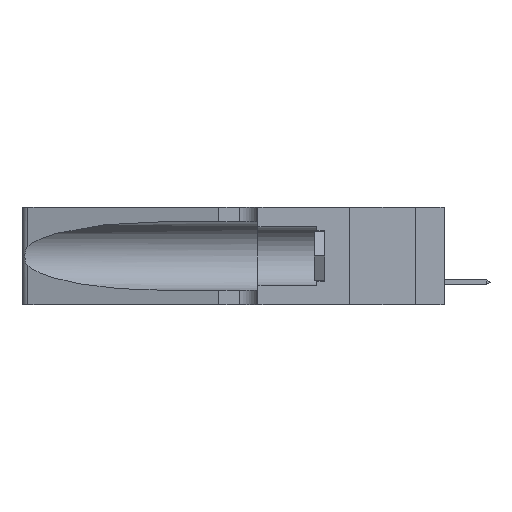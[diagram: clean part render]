
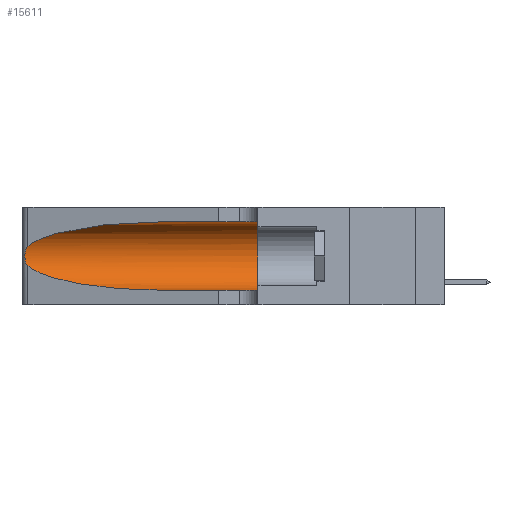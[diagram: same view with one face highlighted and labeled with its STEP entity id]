
A CAD part, left-side view. The second image highlights one B-rep face of the part: STEP entity #15611.
In plain terms, the highlighted cylindrical face has radius 3.308 mm (diameter 6.617 mm), a partial arc.
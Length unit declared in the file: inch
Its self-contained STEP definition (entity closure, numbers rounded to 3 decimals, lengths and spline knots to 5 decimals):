
#83 = B_SPLINE_CURVE_WITH_KNOTS ( 'NONE', 3,
 ( #15689, #11166, #17292, #9687, #17689, #11497, #3763, #14531, #15977, #2344, #2477, #9822, #13083, #13143 ),
 .UNSPECIFIED., .F., .F.,
 ( 4, 2, 2, 2, 2, 2, 4 ),
 ( 0., 0.00027, 0.00053, 0.00107, 0.0016, 0.00187, 0.00214 ),
 .UNSPECIFIED. ) ;
#306 = EDGE_CURVE ( 'NONE', #17060, #13026, #18665, .T. ) ;
#445 = LINE ( 'NONE', #8577, #11906 ) ;
#906 = ORIENTED_EDGE ( 'NONE', *, *, #6104, .T. ) ;
#977 = DIRECTION ( 'NONE',  ( 0., -1., 0. ) ) ;
#1337 = DIRECTION ( 'NONE',  ( 0., 1., 0. ) ) ;
#1874 = EDGE_CURVE ( 'NONE', #13601, #13559, #445, .T. ) ;
#2181 = VECTOR ( 'NONE', #18388, 39.37008 ) ;
#2231 = CIRCLE ( 'NONE', #17281, 0.13025 ) ;
#2344 = CARTESIAN_POINT ( 'NONE',  ( 0.25856, 1.23593, 0.16098 ) ) ;
#2477 = CARTESIAN_POINT ( 'NONE',  ( 0.25789, 1.23486, 0.15765 ) ) ;
#2861 = DIRECTION ( 'NONE',  ( 0., 0., 1. ) ) ;
#3026 =( BOUNDED_CURVE ( )  B_SPLINE_CURVE ( 3, ( #3247, #9378, #3380, #12407 ),
 .UNSPECIFIED., .F., .T. ) 
 B_SPLINE_CURVE_WITH_KNOTS ( ( 4, 4 ),
 ( 3.44316, 4.71239 ),
 .UNSPECIFIED. ) 
 CURVE ( )  GEOMETRIC_REPRESENTATION_ITEM ( )  RATIONAL_B_SPLINE_CURVE ( ( 1., 0.87, 0.87, 1. ) ) 
 REPRESENTATION_ITEM ( '' )  );
#3247 = CARTESIAN_POINT ( 'NONE',  ( 0.25487, 1.22718, 0.14631 ) ) ;
#3380 = CARTESIAN_POINT ( 'NONE',  ( 0.18966, 0.96281, 0.05475 ) ) ;
#3763 = CARTESIAN_POINT ( 'NONE',  ( 0.26075, 1.23896, 0.19203 ) ) ;
#4534 = CARTESIAN_POINT ( 'NONE',  ( 0.1305, 1.61858, 0.31525 ) ) ;
#5158 = EDGE_CURVE ( 'NONE', #13026, #13559, #2231, .T. ) ;
#5350 = CARTESIAN_POINT ( 'NONE',  ( 0.1305, 1.61858, 0.185 ) ) ;
#6104 = EDGE_CURVE ( 'NONE', #9399, #13601, #3026, .T. ) ;
#6399 = EDGE_CURVE ( 'NONE', #17060, #7415, #15752, .T. ) ;
#6512 = CYLINDRICAL_SURFACE ( 'NONE', #12287, 0.13025 ) ;
#6953 = ORIENTED_EDGE ( 'NONE', *, *, #5158, .F. ) ;
#7166 = ORIENTED_EDGE ( 'NONE', *, *, #10112, .T. ) ;
#7371 = CARTESIAN_POINT ( 'NONE',  ( 0.1305, 0.72297, 0.31525 ) ) ;
#7415 = VERTEX_POINT ( 'NONE', #14975 ) ;
#8577 = CARTESIAN_POINT ( 'NONE',  ( 0.1305, 1.61858, 0.05475 ) ) ;
#8954 = ORIENTED_EDGE ( 'NONE', *, *, #6399, .T. ) ;
#9262 = EDGE_LOOP ( 'NONE', ( #8954, #7166, #906, #17290, #6953, #16224 ) ) ;
#9378 = CARTESIAN_POINT ( 'NONE',  ( 0.2373, 1.15595, 0.08982 ) ) ;
#9399 = VERTEX_POINT ( 'NONE', #15605 ) ;
#9687 = CARTESIAN_POINT ( 'NONE',  ( 0.25787, 1.23484, 0.2124 ) ) ;
#9799 = CARTESIAN_POINT ( 'NONE',  ( 0.18966, 0.96281, 0.31525 ) ) ;
#9822 = CARTESIAN_POINT ( 'NONE',  ( 0.25639, 1.23186, 0.15144 ) ) ;
#10112 = EDGE_CURVE ( 'NONE', #7415, #9399, #83, .T. ) ;
#10599 = CARTESIAN_POINT ( 'NONE',  ( 0.1305, 0.35, 0.185 ) ) ;
#11166 = CARTESIAN_POINT ( 'NONE',  ( 0.25555, 1.22994, 0.2215 ) ) ;
#11497 = CARTESIAN_POINT ( 'NONE',  ( 0.26018, 1.23835, 0.19895 ) ) ;
#11552 = DIRECTION ( 'NONE',  ( 0., -1., 0. ) ) ;
#11618 = CARTESIAN_POINT ( 'NONE',  ( 0.1305, 0.72297, 0.05475 ) ) ;
#11877 = CARTESIAN_POINT ( 'NONE',  ( 0.2373, 1.15595, 0.28018 ) ) ;
#11906 = VECTOR ( 'NONE', #977, 39.37008 ) ;
#12287 = AXIS2_PLACEMENT_3D ( 'NONE', #5350, #11552, #18897 ) ;
#12407 = CARTESIAN_POINT ( 'NONE',  ( 0.1305, 0.72297, 0.05475 ) ) ;
#13026 = VERTEX_POINT ( 'NONE', #18769 ) ;
#13083 = CARTESIAN_POINT ( 'NONE',  ( 0.25555, 1.22993, 0.14849 ) ) ;
#13143 = CARTESIAN_POINT ( 'NONE',  ( 0.25487, 1.22718, 0.14631 ) ) ;
#13559 = VERTEX_POINT ( 'NONE', #17091 ) ;
#13601 = VERTEX_POINT ( 'NONE', #11618 ) ;
#14350 = FACE_OUTER_BOUND ( 'NONE', #9262, .T. ) ;
#14531 = CARTESIAN_POINT ( 'NONE',  ( 0.26075, 1.23896, 0.178 ) ) ;
#14975 = CARTESIAN_POINT ( 'NONE',  ( 0.25487, 1.22718, 0.22369 ) ) ;
#15605 = CARTESIAN_POINT ( 'NONE',  ( 0.25487, 1.22718, 0.14631 ) ) ;
#15611 = ADVANCED_FACE ( 'NONE', ( #14350 ), #6512, .F. ) ;
#15689 = CARTESIAN_POINT ( 'NONE',  ( 0.25487, 1.22718, 0.22369 ) ) ;
#15752 =( BOUNDED_CURVE ( )  B_SPLINE_CURVE ( 3, ( #17940, #9799, #11877, #19029 ),
 .UNSPECIFIED., .F., .T. ) 
 B_SPLINE_CURVE_WITH_KNOTS ( ( 4, 4 ),
 ( 1.5708, 2.84003 ),
 .UNSPECIFIED. ) 
 CURVE ( )  GEOMETRIC_REPRESENTATION_ITEM ( )  RATIONAL_B_SPLINE_CURVE ( ( 1., 0.87, 0.87, 1. ) ) 
 REPRESENTATION_ITEM ( '' )  );
#15977 = CARTESIAN_POINT ( 'NONE',  ( 0.26017, 1.23833, 0.17102 ) ) ;
#16224 = ORIENTED_EDGE ( 'NONE', *, *, #306, .F. ) ;
#17060 = VERTEX_POINT ( 'NONE', #7371 ) ;
#17091 = CARTESIAN_POINT ( 'NONE',  ( 0.1305, 0.35, 0.05475 ) ) ;
#17281 = AXIS2_PLACEMENT_3D ( 'NONE', #10599, #1337, #2861 ) ;
#17290 = ORIENTED_EDGE ( 'NONE', *, *, #1874, .T. ) ;
#17292 = CARTESIAN_POINT ( 'NONE',  ( 0.25639, 1.23184, 0.21858 ) ) ;
#17689 = CARTESIAN_POINT ( 'NONE',  ( 0.25854, 1.2359, 0.20912 ) ) ;
#17940 = CARTESIAN_POINT ( 'NONE',  ( 0.1305, 0.72297, 0.31525 ) ) ;
#18388 = DIRECTION ( 'NONE',  ( 0., -1., 0. ) ) ;
#18665 = LINE ( 'NONE', #4534, #2181 ) ;
#18769 = CARTESIAN_POINT ( 'NONE',  ( 0.1305, 0.35, 0.31525 ) ) ;
#18897 = DIRECTION ( 'NONE',  ( 0., 0., -1. ) ) ;
#19029 = CARTESIAN_POINT ( 'NONE',  ( 0.25487, 1.22718, 0.22369 ) ) ;
